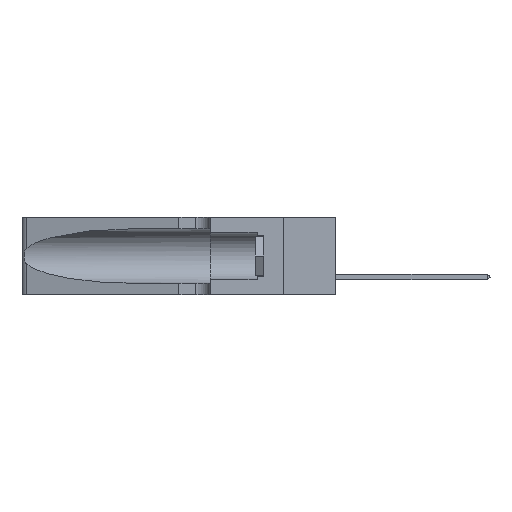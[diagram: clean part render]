
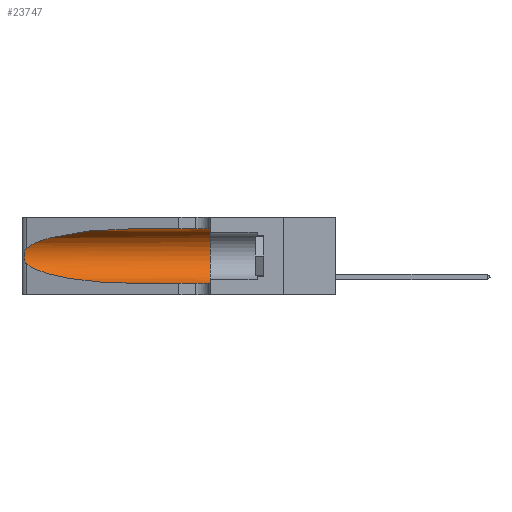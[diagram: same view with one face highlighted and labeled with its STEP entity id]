
A CAD part, left-side view. The second image highlights one B-rep face of the part: STEP entity #23747.
In plain terms, the highlighted cylindrical face has radius 3.308 mm (diameter 6.617 mm), a partial arc.
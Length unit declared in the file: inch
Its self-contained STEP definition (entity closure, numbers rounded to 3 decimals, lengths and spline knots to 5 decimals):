
#460 = EDGE_CURVE ( 'NONE', #9226, #19742, #25578, .T. ) ;
#530 = VERTEX_POINT ( 'NONE', #19887 ) ;
#983 = CARTESIAN_POINT ( 'NONE',  ( 0.25639, 1.23186, 0.15144 ) ) ;
#1081 = CARTESIAN_POINT ( 'NONE',  ( 0.26075, 1.23896, 0.19203 ) ) ;
#1191 = CARTESIAN_POINT ( 'NONE',  ( 0.18966, 0.96281, 0.05475 ) ) ;
#1377 = CARTESIAN_POINT ( 'NONE',  ( 0.1305, 0.72297, 0.05475 ) ) ;
#1562 = CARTESIAN_POINT ( 'NONE',  ( 0.2373, 1.15595, 0.08982 ) ) ;
#2391 = CARTESIAN_POINT ( 'NONE',  ( 0.1305, 0.35, 0.31525 ) ) ;
#2608 = EDGE_CURVE ( 'NONE', #15630, #9226, #4185, .T. ) ;
#2785 = CARTESIAN_POINT ( 'NONE',  ( 0.25787, 1.23484, 0.2124 ) ) ;
#2971 = CARTESIAN_POINT ( 'NONE',  ( 0.25789, 1.23486, 0.15765 ) ) ;
#3059 = CARTESIAN_POINT ( 'NONE',  ( 0.25487, 1.22718, 0.22369 ) ) ;
#3070 = DIRECTION ( 'NONE',  ( 0., -1., 0. ) ) ;
#3498 = CARTESIAN_POINT ( 'NONE',  ( 0.25487, 1.22718, 0.22369 ) ) ;
#3506 = CIRCLE ( 'NONE', #24767, 0.13025 ) ;
#3582 = CARTESIAN_POINT ( 'NONE',  ( 0.1305, 0.72297, 0.31525 ) ) ;
#4185 =( BOUNDED_CURVE ( )  B_SPLINE_CURVE ( 3, ( #3582, #13816, #14064, #3498 ),
 .UNSPECIFIED., .F., .F. ) 
 B_SPLINE_CURVE_WITH_KNOTS ( ( 4, 4 ),
 ( 1.5708, 2.84003 ),
 .UNSPECIFIED. ) 
 CURVE ( )  GEOMETRIC_REPRESENTATION_ITEM ( )  RATIONAL_B_SPLINE_CURVE ( ( 1., 0.87, 0.87, 1. ) ) 
 REPRESENTATION_ITEM ( '' )  );
#4315 = ORIENTED_EDGE ( 'NONE', *, *, #460, .T. ) ;
#4920 = CARTESIAN_POINT ( 'NONE',  ( 0.25856, 1.23593, 0.16098 ) ) ;
#5421 = CARTESIAN_POINT ( 'NONE',  ( 0.1305, 1.61858, 0.05475 ) ) ;
#6973 = CARTESIAN_POINT ( 'NONE',  ( 0.25555, 1.22993, 0.14849 ) ) ;
#7029 = EDGE_CURVE ( 'NONE', #15630, #12887, #25818, .T. ) ;
#7759 = EDGE_CURVE ( 'NONE', #19742, #530, #23198, .T. ) ;
#7989 = ORIENTED_EDGE ( 'NONE', *, *, #2608, .T. ) ;
#9185 = CARTESIAN_POINT ( 'NONE',  ( 0.25487, 1.22718, 0.14631 ) ) ;
#9188 = DIRECTION ( 'NONE',  ( 0., 0., 1. ) ) ;
#9226 = VERTEX_POINT ( 'NONE', #26389 ) ;
#10847 = EDGE_LOOP ( 'NONE', ( #7989, #4315, #26160, #19414, #11688, #26228 ) ) ;
#11231 = CARTESIAN_POINT ( 'NONE',  ( 0.26017, 1.23833, 0.17102 ) ) ;
#11561 = VECTOR ( 'NONE', #21670, 39.37008 ) ;
#11688 = ORIENTED_EDGE ( 'NONE', *, *, #16052, .F. ) ;
#12877 = CYLINDRICAL_SURFACE ( 'NONE', #14982, 0.13025 ) ;
#12887 = VERTEX_POINT ( 'NONE', #2391 ) ;
#13202 = CARTESIAN_POINT ( 'NONE',  ( 0.25555, 1.22994, 0.2215 ) ) ;
#13761 = CARTESIAN_POINT ( 'NONE',  ( 0.25487, 1.22718, 0.14631 ) ) ;
#13808 = DIRECTION ( 'NONE',  ( 0., -1., 0. ) ) ;
#13816 = CARTESIAN_POINT ( 'NONE',  ( 0.18966, 0.96281, 0.31525 ) ) ;
#14064 = CARTESIAN_POINT ( 'NONE',  ( 0.2373, 1.15595, 0.28018 ) ) ;
#14449 = FACE_OUTER_BOUND ( 'NONE', #10847, .T. ) ;
#14979 = CARTESIAN_POINT ( 'NONE',  ( 0.25639, 1.23184, 0.21858 ) ) ;
#14982 = AXIS2_PLACEMENT_3D ( 'NONE', #16975, #13808, #26071 ) ;
#15048 = CARTESIAN_POINT ( 'NONE',  ( 0.1305, 0.35, 0.05475 ) ) ;
#15252 = CARTESIAN_POINT ( 'NONE',  ( 0.1305, 1.61858, 0.31525 ) ) ;
#15630 = VERTEX_POINT ( 'NONE', #18677 ) ;
#16052 = EDGE_CURVE ( 'NONE', #12887, #24310, #3506, .T. ) ;
#16975 = CARTESIAN_POINT ( 'NONE',  ( 0.1305, 1.61858, 0.185 ) ) ;
#17363 = DIRECTION ( 'NONE',  ( 0., 1., 0. ) ) ;
#18131 = CARTESIAN_POINT ( 'NONE',  ( 0.25487, 1.22718, 0.14631 ) ) ;
#18677 = CARTESIAN_POINT ( 'NONE',  ( 0.1305, 0.72297, 0.31525 ) ) ;
#19414 = ORIENTED_EDGE ( 'NONE', *, *, #24381, .T. ) ;
#19742 = VERTEX_POINT ( 'NONE', #18131 ) ;
#19887 = CARTESIAN_POINT ( 'NONE',  ( 0.1305, 0.72297, 0.05475 ) ) ;
#20176 = LINE ( 'NONE', #5421, #11561 ) ;
#20422 = VECTOR ( 'NONE', #3070, 39.37008 ) ;
#21428 = CARTESIAN_POINT ( 'NONE',  ( 0.1305, 0.35, 0.185 ) ) ;
#21670 = DIRECTION ( 'NONE',  ( 0., -1., 0. ) ) ;
#23139 = CARTESIAN_POINT ( 'NONE',  ( 0.25854, 1.2359, 0.20912 ) ) ;
#23198 =( BOUNDED_CURVE ( )  B_SPLINE_CURVE ( 3, ( #13761, #1562, #1191, #1377 ),
 .UNSPECIFIED., .F., .F. ) 
 B_SPLINE_CURVE_WITH_KNOTS ( ( 4, 4 ),
 ( 3.44316, 4.71239 ),
 .UNSPECIFIED. ) 
 CURVE ( )  GEOMETRIC_REPRESENTATION_ITEM ( )  RATIONAL_B_SPLINE_CURVE ( ( 1., 0.87, 0.87, 1. ) ) 
 REPRESENTATION_ITEM ( '' )  );
#23747 = ADVANCED_FACE ( 'NONE', ( #14449 ), #12877, .F. ) ;
#24310 = VERTEX_POINT ( 'NONE', #15048 ) ;
#24381 = EDGE_CURVE ( 'NONE', #530, #24310, #20176, .T. ) ;
#24767 = AXIS2_PLACEMENT_3D ( 'NONE', #21428, #17363, #9188 ) ;
#25125 = CARTESIAN_POINT ( 'NONE',  ( 0.26075, 1.23896, 0.178 ) ) ;
#25483 = CARTESIAN_POINT ( 'NONE',  ( 0.26018, 1.23835, 0.19895 ) ) ;
#25578 = B_SPLINE_CURVE_WITH_KNOTS ( 'NONE', 3,
 ( #3059, #13202, #14979, #2785, #23139, #25483, #1081, #25125, #11231, #4920, #2971, #983, #6973, #9185 ),
 .UNSPECIFIED., .F., .F.,
 ( 4, 2, 2, 2, 2, 2, 4 ),
 ( 0., 0.00027, 0.00053, 0.00107, 0.0016, 0.00187, 0.00214 ),
 .UNSPECIFIED. ) ;
#25818 = LINE ( 'NONE', #15252, #20422 ) ;
#26071 = DIRECTION ( 'NONE',  ( 0., 0., -1. ) ) ;
#26160 = ORIENTED_EDGE ( 'NONE', *, *, #7759, .T. ) ;
#26228 = ORIENTED_EDGE ( 'NONE', *, *, #7029, .F. ) ;
#26389 = CARTESIAN_POINT ( 'NONE',  ( 0.25487, 1.22718, 0.22369 ) ) ;
